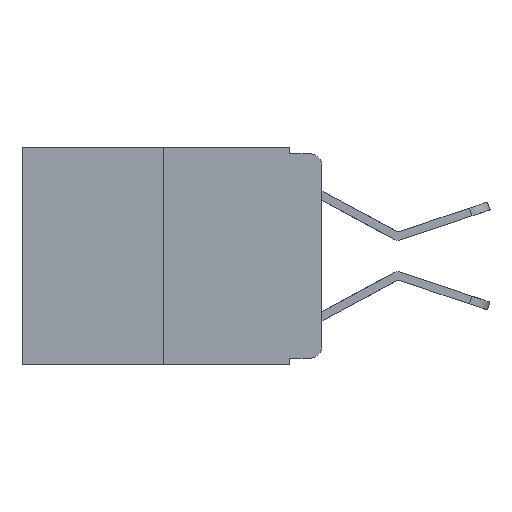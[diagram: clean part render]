
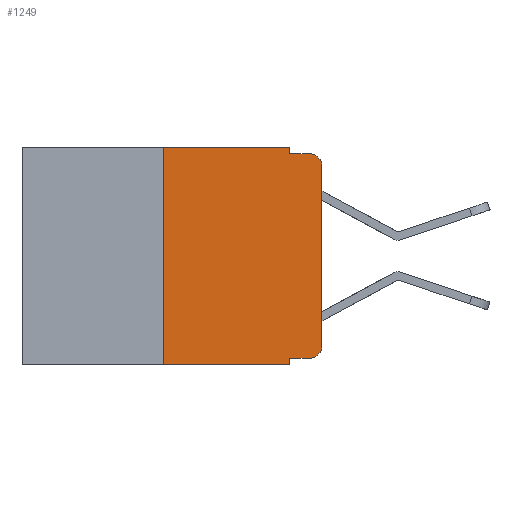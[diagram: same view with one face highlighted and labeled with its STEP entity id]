
A CAD part, left-side view. The second image highlights one B-rep face of the part: STEP entity #1249.
In plain terms, the highlighted planar face has unit normal (-1, 0, 0).
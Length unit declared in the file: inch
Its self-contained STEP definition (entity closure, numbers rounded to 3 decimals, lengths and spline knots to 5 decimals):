
#105 = LINE ( 'NONE', #4077, #12084 ) ;
#151 = ORIENTED_EDGE ( 'NONE', *, *, #15425, .F. ) ;
#206 = DIRECTION ( 'NONE',  ( 0., 0., -1. ) ) ;
#452 = FACE_OUTER_BOUND ( 'NONE', #5558, .T. ) ;
#665 = EDGE_CURVE ( 'NONE', #10024, #11072, #10131, .T. ) ;
#992 = VERTEX_POINT ( 'NONE', #13404 ) ;
#1249 = ADVANCED_FACE ( 'NONE', ( #452 ), #6739, .F. ) ;
#1593 = EDGE_CURVE ( 'NONE', #13721, #10024, #5621, .T. ) ;
#1656 = AXIS2_PLACEMENT_3D ( 'NONE', #11309, #1757, #11235 ) ;
#1674 = ORIENTED_EDGE ( 'NONE', *, *, #665, .T. ) ;
#1757 = DIRECTION ( 'NONE',  ( -1., 0., 0. ) ) ;
#1811 = CARTESIAN_POINT ( 'NONE',  ( 0., 0.051, -0.333 ) ) ;
#1913 = CARTESIAN_POINT ( 'NONE',  ( 0., 0.25, -0.343 ) ) ;
#2219 = CARTESIAN_POINT ( 'NONE',  ( 0., 0.051, 0. ) ) ;
#2237 = LINE ( 'NONE', #3167, #15233 ) ;
#2808 = VECTOR ( 'NONE', #11457, 39.37008 ) ;
#2817 = CARTESIAN_POINT ( 'NONE',  ( 0., 0., -0.03 ) ) ;
#3167 = CARTESIAN_POINT ( 'NONE',  ( 0., 0.473, 0. ) ) ;
#3857 = DIRECTION ( 'NONE',  ( 0., 0., 1. ) ) ;
#3946 = LINE ( 'NONE', #6050, #13101 ) ;
#4077 = CARTESIAN_POINT ( 'NONE',  ( 0., 0.473, -0.343 ) ) ;
#4109 = CARTESIAN_POINT ( 'NONE',  ( 0., 0.051, -0.01 ) ) ;
#4309 = VECTOR ( 'NONE', #3857, 39.37008 ) ;
#4719 = VERTEX_POINT ( 'NONE', #14511 ) ;
#4819 = VERTEX_POINT ( 'NONE', #12274 ) ;
#5238 = CARTESIAN_POINT ( 'NONE',  ( 0., 0.02, -0.313 ) ) ;
#5488 = ORIENTED_EDGE ( 'NONE', *, *, #5867, .F. ) ;
#5558 = EDGE_LOOP ( 'NONE', ( #7426, #1674, #9220, #151, #5488, #15964, #11466, #15530, #16150, #13380 ) ) ;
#5621 = LINE ( 'NONE', #8672, #15133 ) ;
#5775 = LINE ( 'NONE', #1811, #11968 ) ;
#5867 = EDGE_CURVE ( 'NONE', #4819, #11338, #2237, .T. ) ;
#6050 = CARTESIAN_POINT ( 'NONE',  ( 0., 0.051, 0. ) ) ;
#6234 = AXIS2_PLACEMENT_3D ( 'NONE', #10439, #8020, #206 ) ;
#6354 = CARTESIAN_POINT ( 'NONE',  ( 0., 0.25, 0. ) ) ;
#6490 = EDGE_CURVE ( 'NONE', #10909, #4719, #105, .T. ) ;
#6492 = DIRECTION ( 'NONE',  ( 0., 0., -1. ) ) ;
#6739 = PLANE ( 'NONE',  #6234 ) ;
#7313 = DIRECTION ( 'NONE',  ( 0., 0., -1. ) ) ;
#7426 = ORIENTED_EDGE ( 'NONE', *, *, #1593, .T. ) ;
#7518 = AXIS2_PLACEMENT_3D ( 'NONE', #5238, #13906, #6492 ) ;
#7901 = DIRECTION ( 'NONE',  ( 0., -1., 0. ) ) ;
#8020 = DIRECTION ( 'NONE',  ( 1., 0., 0. ) ) ;
#8447 = VECTOR ( 'NONE', #12309, 39.37008 ) ;
#8482 = LINE ( 'NONE', #6354, #4309 ) ;
#8672 = CARTESIAN_POINT ( 'NONE',  ( 0., 0., 0. ) ) ;
#9220 = ORIENTED_EDGE ( 'NONE', *, *, #16250, .F. ) ;
#9812 = CARTESIAN_POINT ( 'NONE',  ( 0., 0.02, -0.01 ) ) ;
#9876 = DIRECTION ( 'NONE',  ( 0., 0., 1. ) ) ;
#10024 = VERTEX_POINT ( 'NONE', #2817 ) ;
#10131 = CIRCLE ( 'NONE', #1656, 0.02 ) ;
#10203 = CARTESIAN_POINT ( 'NONE',  ( 0., 0.051, -0.01 ) ) ;
#10355 = CARTESIAN_POINT ( 'NONE',  ( 0., 0.051, 0. ) ) ;
#10439 = CARTESIAN_POINT ( 'NONE',  ( 0., 0.473, 0. ) ) ;
#10694 = VERTEX_POINT ( 'NONE', #15355 ) ;
#10909 = VERTEX_POINT ( 'NONE', #1913 ) ;
#11072 = VERTEX_POINT ( 'NONE', #9812 ) ;
#11235 = DIRECTION ( 'NONE',  ( 0., 0., -1. ) ) ;
#11309 = CARTESIAN_POINT ( 'NONE',  ( 0., 0.02, -0.03 ) ) ;
#11338 = VERTEX_POINT ( 'NONE', #10355 ) ;
#11457 = DIRECTION ( 'NONE',  ( 0., -1., 0. ) ) ;
#11466 = ORIENTED_EDGE ( 'NONE', *, *, #6490, .T. ) ;
#11925 = DIRECTION ( 'NONE',  ( 0., -1., 0. ) ) ;
#11968 = VECTOR ( 'NONE', #11925, 39.37008 ) ;
#12000 = CIRCLE ( 'NONE', #7518, 0.02 ) ;
#12073 = EDGE_CURVE ( 'NONE', #10694, #13721, #12000, .T. ) ;
#12084 = VECTOR ( 'NONE', #7901, 39.37008 ) ;
#12274 = CARTESIAN_POINT ( 'NONE',  ( 0., 0.25, 0. ) ) ;
#12309 = DIRECTION ( 'NONE',  ( 0., 0., -1. ) ) ;
#12464 = LINE ( 'NONE', #2219, #8447 ) ;
#12819 = LINE ( 'NONE', #10203, #2808 ) ;
#12902 = EDGE_CURVE ( 'NONE', #992, #10694, #5775, .T. ) ;
#13101 = VECTOR ( 'NONE', #7313, 39.37008 ) ;
#13380 = ORIENTED_EDGE ( 'NONE', *, *, #12073, .T. ) ;
#13404 = CARTESIAN_POINT ( 'NONE',  ( 0., 0.051, -0.333 ) ) ;
#13420 = CARTESIAN_POINT ( 'NONE',  ( 0., 0., -0.313 ) ) ;
#13428 = VERTEX_POINT ( 'NONE', #4109 ) ;
#13721 = VERTEX_POINT ( 'NONE', #13420 ) ;
#13747 = EDGE_CURVE ( 'NONE', #992, #4719, #3946, .T. ) ;
#13906 = DIRECTION ( 'NONE',  ( -1., 0., 0. ) ) ;
#14373 = DIRECTION ( 'NONE',  ( 0., -1., 0. ) ) ;
#14511 = CARTESIAN_POINT ( 'NONE',  ( 0., 0.051, -0.343 ) ) ;
#14568 = EDGE_CURVE ( 'NONE', #10909, #4819, #8482, .T. ) ;
#15133 = VECTOR ( 'NONE', #9876, 39.37008 ) ;
#15233 = VECTOR ( 'NONE', #14373, 39.37008 ) ;
#15355 = CARTESIAN_POINT ( 'NONE',  ( 0., 0.02, -0.333 ) ) ;
#15425 = EDGE_CURVE ( 'NONE', #11338, #13428, #12464, .T. ) ;
#15530 = ORIENTED_EDGE ( 'NONE', *, *, #13747, .F. ) ;
#15964 = ORIENTED_EDGE ( 'NONE', *, *, #14568, .F. ) ;
#16150 = ORIENTED_EDGE ( 'NONE', *, *, #12902, .T. ) ;
#16250 = EDGE_CURVE ( 'NONE', #13428, #11072, #12819, .T. ) ;
